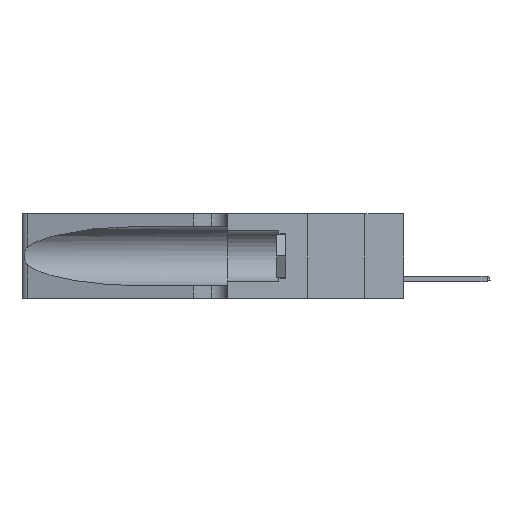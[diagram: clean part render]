
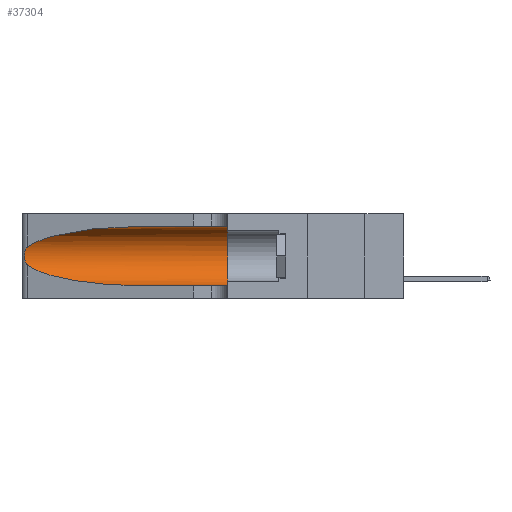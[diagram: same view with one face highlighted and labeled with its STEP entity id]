
A CAD part, left-side view. The second image highlights one B-rep face of the part: STEP entity #37304.
In plain terms, the highlighted cylindrical face has radius 3.308 mm (diameter 6.617 mm), a partial arc.
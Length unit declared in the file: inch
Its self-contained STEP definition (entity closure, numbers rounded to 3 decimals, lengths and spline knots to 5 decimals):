
#580 = CARTESIAN_POINT ( 'NONE',  ( 0.25854, 1.2359, 0.20912 ) ) ;
#2563 = DIRECTION ( 'NONE',  ( 0., 0., 1. ) ) ;
#2873 = DIRECTION ( 'NONE',  ( 0., -1., 0. ) ) ;
#2988 = EDGE_CURVE ( 'NONE', #12721, #26967, #27244, .T. ) ;
#3769 = CARTESIAN_POINT ( 'NONE',  ( 0.1305, 1.61858, 0.05475 ) ) ;
#3913 = DIRECTION ( 'NONE',  ( 0., -1., 0. ) ) ;
#4559 = LINE ( 'NONE', #3769, #44453 ) ;
#8539 = CARTESIAN_POINT ( 'NONE',  ( 0.26018, 1.23835, 0.19895 ) ) ;
#8698 = CARTESIAN_POINT ( 'NONE',  ( 0.25639, 1.23186, 0.15144 ) ) ;
#10135 = CARTESIAN_POINT ( 'NONE',  ( 0.25487, 1.22718, 0.22369 ) ) ;
#11161 = AXIS2_PLACEMENT_3D ( 'NONE', #11859, #13348, #26001 ) ;
#11859 = CARTESIAN_POINT ( 'NONE',  ( 0.1305, 1.61858, 0.185 ) ) ;
#12422 = CARTESIAN_POINT ( 'NONE',  ( 0.25487, 1.22718, 0.22369 ) ) ;
#12580 = CARTESIAN_POINT ( 'NONE',  ( 0.25487, 1.22718, 0.14631 ) ) ;
#12721 = VERTEX_POINT ( 'NONE', #46736 ) ;
#13348 = DIRECTION ( 'NONE',  ( 0., -1., 0. ) ) ;
#13683 = CARTESIAN_POINT ( 'NONE',  ( 0.2373, 1.15595, 0.28018 ) ) ;
#14520 = CARTESIAN_POINT ( 'NONE',  ( 0.25487, 1.22718, 0.14631 ) ) ;
#14902 = ORIENTED_EDGE ( 'NONE', *, *, #41274, .T. ) ;
#16300 = CARTESIAN_POINT ( 'NONE',  ( 0.26075, 1.23896, 0.178 ) ) ;
#16354 = CARTESIAN_POINT ( 'NONE',  ( 0.1305, 0.72297, 0.05475 ) ) ;
#16798 = CARTESIAN_POINT ( 'NONE',  ( 0.2373, 1.15595, 0.08982 ) ) ;
#17734 = EDGE_CURVE ( 'NONE', #38458, #12721, #36253, .T. ) ;
#18011 = CIRCLE ( 'NONE', #40894, 0.13025 ) ;
#18444 = CYLINDRICAL_SURFACE ( 'NONE', #11161, 0.13025 ) ;
#19837 = CARTESIAN_POINT ( 'NONE',  ( 0.25639, 1.23184, 0.21858 ) ) ;
#20609 = VERTEX_POINT ( 'NONE', #16354 ) ;
#20732 = CARTESIAN_POINT ( 'NONE',  ( 0.1305, 0.72297, 0.31525 ) ) ;
#22253 = CARTESIAN_POINT ( 'NONE',  ( 0.1305, 1.61858, 0.31525 ) ) ;
#24011 = CARTESIAN_POINT ( 'NONE',  ( 0.25856, 1.23593, 0.16098 ) ) ;
#24581 = ORIENTED_EDGE ( 'NONE', *, *, #42533, .T. ) ;
#25050 = CARTESIAN_POINT ( 'NONE',  ( 0.1305, 0.35, 0.31525 ) ) ;
#26001 = DIRECTION ( 'NONE',  ( 0., 0., -1. ) ) ;
#26879 = CARTESIAN_POINT ( 'NONE',  ( 0.1305, 0.72297, 0.31525 ) ) ;
#26967 = VERTEX_POINT ( 'NONE', #14520 ) ;
#27244 = B_SPLINE_CURVE_WITH_KNOTS ( 'NONE', 3,
 ( #12422, #42996, #19837, #27755, #580, #8539, #35565, #16300, #43302, #24011, #27922, #8698, #39598, #12580 ),
 .UNSPECIFIED., .F., .F.,
 ( 4, 2, 2, 2, 2, 2, 4 ),
 ( 0., 0.00027, 0.00053, 0.00107, 0.0016, 0.00187, 0.00214 ),
 .UNSPECIFIED. ) ;
#27755 = CARTESIAN_POINT ( 'NONE',  ( 0.25787, 1.23484, 0.2124 ) ) ;
#27922 = CARTESIAN_POINT ( 'NONE',  ( 0.25789, 1.23486, 0.15765 ) ) ;
#30219 = CARTESIAN_POINT ( 'NONE',  ( 0.1305, 0.35, 0.05475 ) ) ;
#32837 = VERTEX_POINT ( 'NONE', #25050 ) ;
#33248 = ORIENTED_EDGE ( 'NONE', *, *, #47434, .F. ) ;
#34081 = VERTEX_POINT ( 'NONE', #30219 ) ;
#34547 = VECTOR ( 'NONE', #2873, 39.37008 ) ;
#35565 = CARTESIAN_POINT ( 'NONE',  ( 0.26075, 1.23896, 0.19203 ) ) ;
#36253 =( BOUNDED_CURVE ( )  B_SPLINE_CURVE ( 3, ( #20732, #36289, #13683, #10135 ),
 .UNSPECIFIED., .F., .F. ) 
 B_SPLINE_CURVE_WITH_KNOTS ( ( 4, 4 ),
 ( 1.5708, 2.84003 ),
 .UNSPECIFIED. ) 
 CURVE ( )  GEOMETRIC_REPRESENTATION_ITEM ( )  RATIONAL_B_SPLINE_CURVE ( ( 1., 0.87, 0.87, 1. ) ) 
 REPRESENTATION_ITEM ( '' )  );
#36289 = CARTESIAN_POINT ( 'NONE',  ( 0.18966, 0.96281, 0.31525 ) ) ;
#37304 = ADVANCED_FACE ( 'NONE', ( #38371 ), #18444, .F. ) ;
#38371 = FACE_OUTER_BOUND ( 'NONE', #40401, .T. ) ;
#38458 = VERTEX_POINT ( 'NONE', #26879 ) ;
#39598 = CARTESIAN_POINT ( 'NONE',  ( 0.25555, 1.22993, 0.14849 ) ) ;
#40118 = CARTESIAN_POINT ( 'NONE',  ( 0.18966, 0.96281, 0.05475 ) ) ;
#40401 = EDGE_LOOP ( 'NONE', ( #46239, #47384, #14902, #24581, #33248, #49778 ) ) ;
#40894 = AXIS2_PLACEMENT_3D ( 'NONE', #48796, #41249, #2563 ) ;
#41249 = DIRECTION ( 'NONE',  ( 0., 1., 0. ) ) ;
#41274 = EDGE_CURVE ( 'NONE', #26967, #20609, #41580, .T. ) ;
#41580 =( BOUNDED_CURVE ( )  B_SPLINE_CURVE ( 3, ( #47637, #16798, #40118, #43785 ),
 .UNSPECIFIED., .F., .F. ) 
 B_SPLINE_CURVE_WITH_KNOTS ( ( 4, 4 ),
 ( 3.44316, 4.71239 ),
 .UNSPECIFIED. ) 
 CURVE ( )  GEOMETRIC_REPRESENTATION_ITEM ( )  RATIONAL_B_SPLINE_CURVE ( ( 1., 0.87, 0.87, 1. ) ) 
 REPRESENTATION_ITEM ( '' )  );
#42533 = EDGE_CURVE ( 'NONE', #20609, #34081, #4559, .T. ) ;
#42996 = CARTESIAN_POINT ( 'NONE',  ( 0.25555, 1.22994, 0.2215 ) ) ;
#43302 = CARTESIAN_POINT ( 'NONE',  ( 0.26017, 1.23833, 0.17102 ) ) ;
#43785 = CARTESIAN_POINT ( 'NONE',  ( 0.1305, 0.72297, 0.05475 ) ) ;
#44453 = VECTOR ( 'NONE', #3913, 39.37008 ) ;
#44749 = LINE ( 'NONE', #22253, #34547 ) ;
#45990 = EDGE_CURVE ( 'NONE', #38458, #32837, #44749, .T. ) ;
#46239 = ORIENTED_EDGE ( 'NONE', *, *, #17734, .T. ) ;
#46736 = CARTESIAN_POINT ( 'NONE',  ( 0.25487, 1.22718, 0.22369 ) ) ;
#47384 = ORIENTED_EDGE ( 'NONE', *, *, #2988, .T. ) ;
#47434 = EDGE_CURVE ( 'NONE', #32837, #34081, #18011, .T. ) ;
#47637 = CARTESIAN_POINT ( 'NONE',  ( 0.25487, 1.22718, 0.14631 ) ) ;
#48796 = CARTESIAN_POINT ( 'NONE',  ( 0.1305, 0.35, 0.185 ) ) ;
#49778 = ORIENTED_EDGE ( 'NONE', *, *, #45990, .F. ) ;
